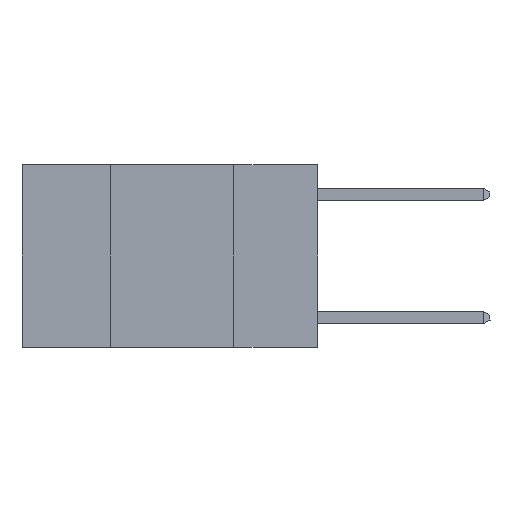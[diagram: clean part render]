
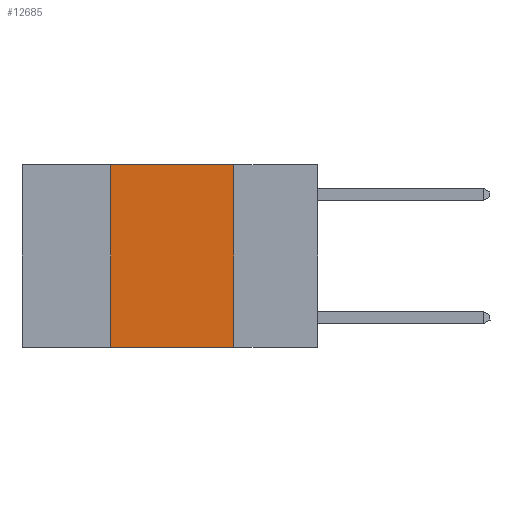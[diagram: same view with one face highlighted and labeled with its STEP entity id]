
A CAD part, left-side view. The second image highlights one B-rep face of the part: STEP entity #12685.
In plain terms, the highlighted planar face has unit normal (-1, 0, 0).
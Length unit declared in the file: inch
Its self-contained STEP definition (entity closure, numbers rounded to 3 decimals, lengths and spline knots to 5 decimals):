
#841 = DIRECTION ( 'NONE',  ( 0., -1., 0. ) ) ;
#1395 = CARTESIAN_POINT ( 'NONE',  ( 0., 0.42, 0. ) ) ;
#1504 = DIRECTION ( 'NONE',  ( 0., 0., 1. ) ) ;
#3442 = PLANE ( 'NONE',  #13234 ) ;
#3564 = CARTESIAN_POINT ( 'NONE',  ( 0., 0.6, -0.37 ) ) ;
#5049 = CARTESIAN_POINT ( 'NONE',  ( 0., 0.17, 0. ) ) ;
#5285 = DIRECTION ( 'NONE',  ( 1., 0., 0. ) ) ;
#5415 = DIRECTION ( 'NONE',  ( 0., -1., 0. ) ) ;
#5423 = LINE ( 'NONE', #5049, #19433 ) ;
#6712 = FACE_OUTER_BOUND ( 'NONE', #16006, .T. ) ;
#8092 = VERTEX_POINT ( 'NONE', #15205 ) ;
#8914 = CARTESIAN_POINT ( 'NONE',  ( 0., 0.17, 0. ) ) ;
#9057 = EDGE_CURVE ( 'NONE', #8092, #11729, #17445, .T. ) ;
#10463 = ORIENTED_EDGE ( 'NONE', *, *, #20787, .F. ) ;
#11729 = VERTEX_POINT ( 'NONE', #15182 ) ;
#11843 = CARTESIAN_POINT ( 'NONE',  ( 0., 0.6, 0. ) ) ;
#12417 = CARTESIAN_POINT ( 'NONE',  ( 0., 0.42, 0. ) ) ;
#12685 = ADVANCED_FACE ( 'NONE', ( #6712 ), #3442, .F. ) ;
#13148 = VECTOR ( 'NONE', #5415, 39.37008 ) ;
#13234 = AXIS2_PLACEMENT_3D ( 'NONE', #16249, #5285, #18091 ) ;
#13548 = ORIENTED_EDGE ( 'NONE', *, *, #16348, .F. ) ;
#14126 = ORIENTED_EDGE ( 'NONE', *, *, #16401, .F. ) ;
#15182 = CARTESIAN_POINT ( 'NONE',  ( 0., 0.17, -0.37 ) ) ;
#15205 = CARTESIAN_POINT ( 'NONE',  ( 0., 0.42, -0.37 ) ) ;
#15280 = VECTOR ( 'NONE', #841, 39.37008 ) ;
#16006 = EDGE_LOOP ( 'NONE', ( #13548, #10463, #14126, #18402 ) ) ;
#16249 = CARTESIAN_POINT ( 'NONE',  ( 0., 0.6, 0. ) ) ;
#16348 = EDGE_CURVE ( 'NONE', #22981, #11729, #5423, .T. ) ;
#16401 = EDGE_CURVE ( 'NONE', #8092, #19190, #23025, .T. ) ;
#17445 = LINE ( 'NONE', #3564, #13148 ) ;
#18091 = DIRECTION ( 'NONE',  ( 0., 0., -1. ) ) ;
#18306 = VECTOR ( 'NONE', #1504, 39.37008 ) ;
#18402 = ORIENTED_EDGE ( 'NONE', *, *, #9057, .T. ) ;
#19190 = VERTEX_POINT ( 'NONE', #1395 ) ;
#19433 = VECTOR ( 'NONE', #19674, 39.37008 ) ;
#19524 = LINE ( 'NONE', #11843, #15280 ) ;
#19674 = DIRECTION ( 'NONE',  ( 0., 0., -1. ) ) ;
#20787 = EDGE_CURVE ( 'NONE', #19190, #22981, #19524, .T. ) ;
#22981 = VERTEX_POINT ( 'NONE', #8914 ) ;
#23025 = LINE ( 'NONE', #12417, #18306 ) ;
